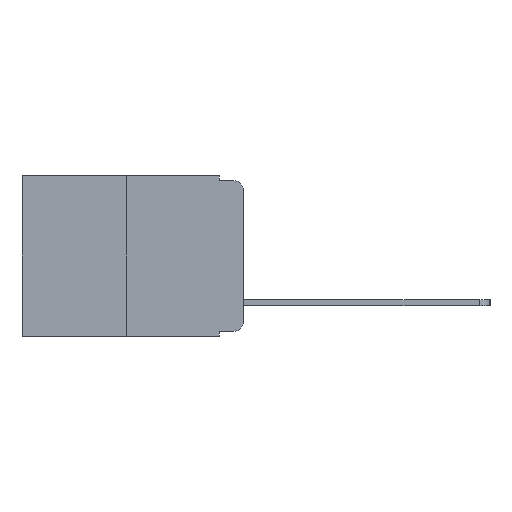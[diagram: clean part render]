
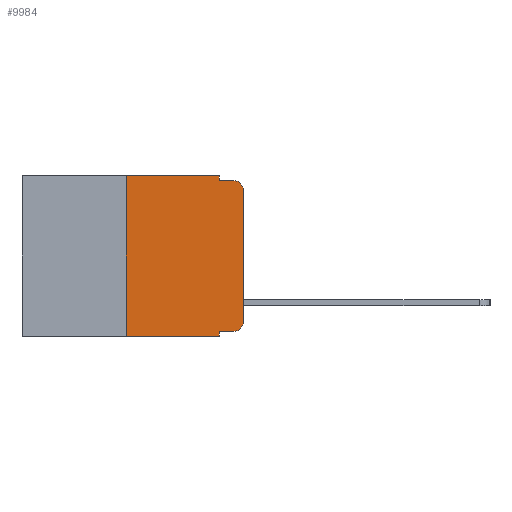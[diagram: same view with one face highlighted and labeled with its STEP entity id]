
A CAD part, left-side view. The second image highlights one B-rep face of the part: STEP entity #9984.
In plain terms, the highlighted planar face has unit normal (-1, 0, 0).
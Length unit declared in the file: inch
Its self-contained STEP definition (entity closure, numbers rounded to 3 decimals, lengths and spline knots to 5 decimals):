
#122 = CIRCLE ( 'NONE', #6206, 0.02 ) ;
#164 = ORIENTED_EDGE ( 'NONE', *, *, #8405, .T. ) ;
#205 = EDGE_CURVE ( 'NONE', #3991, #4920, #3338, .T. ) ;
#240 = LINE ( 'NONE', #12074, #12665 ) ;
#513 = CARTESIAN_POINT ( 'NONE',  ( 0., 0.473, 0. ) ) ;
#570 = ORIENTED_EDGE ( 'NONE', *, *, #628, .F. ) ;
#573 = DIRECTION ( 'NONE',  ( 0., -1., 0. ) ) ;
#597 = CARTESIAN_POINT ( 'NONE',  ( 0., 0.051, 0. ) ) ;
#601 = CARTESIAN_POINT ( 'NONE',  ( 0., 0.02, -0.03 ) ) ;
#628 = EDGE_CURVE ( 'NONE', #4920, #9692, #10298, .T. ) ;
#677 = CARTESIAN_POINT ( 'NONE',  ( 0., 0., -0.03 ) ) ;
#691 = CARTESIAN_POINT ( 'NONE',  ( 0., 0.051, -0.333 ) ) ;
#701 = DIRECTION ( 'NONE',  ( 0., -1., 0. ) ) ;
#723 = VERTEX_POINT ( 'NONE', #11103 ) ;
#908 = CARTESIAN_POINT ( 'NONE',  ( 0., 0.02, -0.01 ) ) ;
#939 = CARTESIAN_POINT ( 'NONE',  ( 0., 0.25, 0. ) ) ;
#1399 = ORIENTED_EDGE ( 'NONE', *, *, #7241, .T. ) ;
#1420 = CARTESIAN_POINT ( 'NONE',  ( 0., 0.473, 0. ) ) ;
#1516 = DIRECTION ( 'NONE',  ( 0., -1., 0. ) ) ;
#1553 = CARTESIAN_POINT ( 'NONE',  ( 0., 0.051, 0. ) ) ;
#1816 = DIRECTION ( 'NONE',  ( 0., 0., -1. ) ) ;
#2101 = LINE ( 'NONE', #7983, #6909 ) ;
#2415 = DIRECTION ( 'NONE',  ( 0., 0., -1. ) ) ;
#2468 = CARTESIAN_POINT ( 'NONE',  ( 0., 0.473, -0.343 ) ) ;
#2479 = EDGE_CURVE ( 'NONE', #2887, #10486, #5173, .T. ) ;
#2554 = DIRECTION ( 'NONE',  ( 0., 0., -1. ) ) ;
#2562 = CARTESIAN_POINT ( 'NONE',  ( 0., 0.02, -0.313 ) ) ;
#2796 = LINE ( 'NONE', #6590, #8195 ) ;
#2887 = VERTEX_POINT ( 'NONE', #8451 ) ;
#2925 = VERTEX_POINT ( 'NONE', #677 ) ;
#3108 = ORIENTED_EDGE ( 'NONE', *, *, #6479, .F. ) ;
#3338 = LINE ( 'NONE', #513, #8112 ) ;
#3464 = CARTESIAN_POINT ( 'NONE',  ( 0., 0., -0.313 ) ) ;
#3470 = EDGE_CURVE ( 'NONE', #11506, #3991, #240, .T. ) ;
#3555 = DIRECTION ( 'NONE',  ( 0., 0., -1. ) ) ;
#3897 = CARTESIAN_POINT ( 'NONE',  ( 0., 0.051, -0.01 ) ) ;
#3991 = VERTEX_POINT ( 'NONE', #939 ) ;
#4037 = ORIENTED_EDGE ( 'NONE', *, *, #5660, .F. ) ;
#4115 = EDGE_CURVE ( 'NONE', #12175, #2925, #2101, .T. ) ;
#4289 = EDGE_CURVE ( 'NONE', #10486, #12175, #7353, .T. ) ;
#4512 = EDGE_LOOP ( 'NONE', ( #10390, #164, #3108, #570, #8482, #6254, #1399, #4037, #9075, #11562 ) ) ;
#4920 = VERTEX_POINT ( 'NONE', #1553 ) ;
#5173 = LINE ( 'NONE', #691, #12688 ) ;
#5392 = CARTESIAN_POINT ( 'NONE',  ( 0., 0.051, 0. ) ) ;
#5660 = EDGE_CURVE ( 'NONE', #2887, #723, #10579, .T. ) ;
#6057 = FACE_OUTER_BOUND ( 'NONE', #4512, .T. ) ;
#6206 = AXIS2_PLACEMENT_3D ( 'NONE', #601, #7578, #1816 ) ;
#6254 = ORIENTED_EDGE ( 'NONE', *, *, #3470, .F. ) ;
#6378 = LINE ( 'NONE', #2468, #8617 ) ;
#6479 = EDGE_CURVE ( 'NONE', #9692, #12466, #2796, .T. ) ;
#6590 = CARTESIAN_POINT ( 'NONE',  ( 0., 0.051, -0.01 ) ) ;
#6658 = DIRECTION ( 'NONE',  ( 0., -1., 0. ) ) ;
#6909 = VECTOR ( 'NONE', #9888, 39.37008 ) ;
#7213 = PLANE ( 'NONE',  #10107 ) ;
#7241 = EDGE_CURVE ( 'NONE', #11506, #723, #6378, .T. ) ;
#7353 = CIRCLE ( 'NONE', #10776, 0.02 ) ;
#7578 = DIRECTION ( 'NONE',  ( -1., 0., 0. ) ) ;
#7781 = VECTOR ( 'NONE', #10135, 39.37008 ) ;
#7802 = VECTOR ( 'NONE', #2554, 39.37008 ) ;
#7875 = CARTESIAN_POINT ( 'NONE',  ( 0., 0.25, -0.343 ) ) ;
#7983 = CARTESIAN_POINT ( 'NONE',  ( 0., 0., 0. ) ) ;
#8112 = VECTOR ( 'NONE', #701, 39.37008 ) ;
#8161 = DIRECTION ( 'NONE',  ( 1., 0., 0. ) ) ;
#8195 = VECTOR ( 'NONE', #573, 39.37008 ) ;
#8320 = DIRECTION ( 'NONE',  ( 0., 0., 1. ) ) ;
#8405 = EDGE_CURVE ( 'NONE', #2925, #12466, #122, .T. ) ;
#8451 = CARTESIAN_POINT ( 'NONE',  ( 0., 0.051, -0.333 ) ) ;
#8482 = ORIENTED_EDGE ( 'NONE', *, *, #205, .F. ) ;
#8617 = VECTOR ( 'NONE', #1516, 39.37008 ) ;
#9035 = CARTESIAN_POINT ( 'NONE',  ( 0., 0.02, -0.333 ) ) ;
#9075 = ORIENTED_EDGE ( 'NONE', *, *, #2479, .T. ) ;
#9250 = DIRECTION ( 'NONE',  ( -1., 0., 0. ) ) ;
#9692 = VERTEX_POINT ( 'NONE', #3897 ) ;
#9888 = DIRECTION ( 'NONE',  ( 0., 0., 1. ) ) ;
#9984 = ADVANCED_FACE ( 'NONE', ( #6057 ), #7213, .F. ) ;
#10107 = AXIS2_PLACEMENT_3D ( 'NONE', #1420, #8161, #2415 ) ;
#10135 = DIRECTION ( 'NONE',  ( 0., 0., -1. ) ) ;
#10298 = LINE ( 'NONE', #597, #7802 ) ;
#10390 = ORIENTED_EDGE ( 'NONE', *, *, #4115, .T. ) ;
#10486 = VERTEX_POINT ( 'NONE', #9035 ) ;
#10579 = LINE ( 'NONE', #5392, #7781 ) ;
#10776 = AXIS2_PLACEMENT_3D ( 'NONE', #2562, #9250, #3555 ) ;
#11103 = CARTESIAN_POINT ( 'NONE',  ( 0., 0.051, -0.343 ) ) ;
#11506 = VERTEX_POINT ( 'NONE', #7875 ) ;
#11562 = ORIENTED_EDGE ( 'NONE', *, *, #4289, .T. ) ;
#12074 = CARTESIAN_POINT ( 'NONE',  ( 0., 0.25, 0. ) ) ;
#12175 = VERTEX_POINT ( 'NONE', #3464 ) ;
#12466 = VERTEX_POINT ( 'NONE', #908 ) ;
#12665 = VECTOR ( 'NONE', #8320, 39.37008 ) ;
#12688 = VECTOR ( 'NONE', #6658, 39.37008 ) ;
